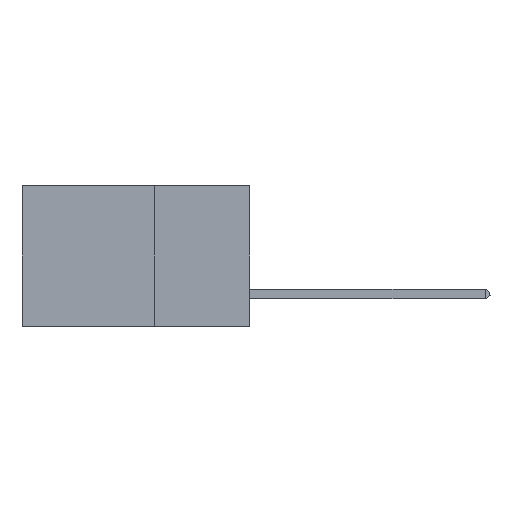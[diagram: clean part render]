
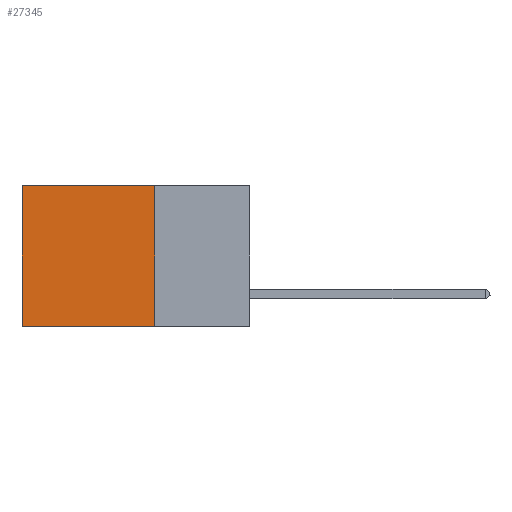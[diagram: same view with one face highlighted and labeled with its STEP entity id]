
A CAD part, left-side view. The second image highlights one B-rep face of the part: STEP entity #27345.
In plain terms, the highlighted planar face has unit normal (-1, 0, 0).
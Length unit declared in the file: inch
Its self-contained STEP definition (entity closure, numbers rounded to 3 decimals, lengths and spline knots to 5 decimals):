
#3004 = EDGE_CURVE ( 'NONE', #25553, #34495, #31278, .T. ) ;
#9082 = ORIENTED_EDGE ( 'NONE', *, *, #22281, .T. ) ;
#9734 = CARTESIAN_POINT ( 'NONE',  ( 0.2875, 0.25, 0. ) ) ;
#10029 = ORIENTED_EDGE ( 'NONE', *, *, #27524, .T. ) ;
#12877 = FACE_OUTER_BOUND ( 'NONE', #13228, .T. ) ;
#13228 = EDGE_LOOP ( 'NONE', ( #10029, #34841, #28919, #9082 ) ) ;
#13406 = VECTOR ( 'NONE', #40061, 39.37008 ) ;
#14698 = CARTESIAN_POINT ( 'NONE',  ( 0.2875, 0.25, -0.37 ) ) ;
#17171 = CARTESIAN_POINT ( 'NONE',  ( 0.2875, 0.6, -0.37 ) ) ;
#20604 = DIRECTION ( 'NONE',  ( 0., 1., 0. ) ) ;
#22114 = VECTOR ( 'NONE', #20604, 39.37008 ) ;
#22281 = EDGE_CURVE ( 'NONE', #36832, #34794, #28862, .T. ) ;
#22509 = LINE ( 'NONE', #36580, #13406 ) ;
#23322 = CARTESIAN_POINT ( 'NONE',  ( 0.2875, 0.25, -0.37 ) ) ;
#23557 = DIRECTION ( 'NONE',  ( 0., 1., 0. ) ) ;
#24412 = LINE ( 'NONE', #42494, #33559 ) ;
#25553 = VERTEX_POINT ( 'NONE', #14698 ) ;
#26775 = VECTOR ( 'NONE', #23557, 39.37008 ) ;
#27345 = ADVANCED_FACE ( 'NONE', ( #12877 ), #30386, .F. ) ;
#27524 = EDGE_CURVE ( 'NONE', #34794, #34495, #22509, .T. ) ;
#28862 = LINE ( 'NONE', #30308, #26775 ) ;
#28919 = ORIENTED_EDGE ( 'NONE', *, *, #34675, .F. ) ;
#29230 = AXIS2_PLACEMENT_3D ( 'NONE', #40011, #43619, #37605 ) ;
#29430 = CARTESIAN_POINT ( 'NONE',  ( 0.2875, 0.6, 0. ) ) ;
#30308 = CARTESIAN_POINT ( 'NONE',  ( 0.2875, 0.25, 0. ) ) ;
#30386 = PLANE ( 'NONE',  #29230 ) ;
#31278 = LINE ( 'NONE', #23322, #22114 ) ;
#32252 = DIRECTION ( 'NONE',  ( 0., 0., -1. ) ) ;
#33559 = VECTOR ( 'NONE', #32252, 39.37008 ) ;
#34495 = VERTEX_POINT ( 'NONE', #17171 ) ;
#34675 = EDGE_CURVE ( 'NONE', #36832, #25553, #24412, .T. ) ;
#34794 = VERTEX_POINT ( 'NONE', #29430 ) ;
#34841 = ORIENTED_EDGE ( 'NONE', *, *, #3004, .F. ) ;
#36580 = CARTESIAN_POINT ( 'NONE',  ( 0.2875, 0.6, 0. ) ) ;
#36832 = VERTEX_POINT ( 'NONE', #9734 ) ;
#37605 = DIRECTION ( 'NONE',  ( 0., 0., -1. ) ) ;
#40011 = CARTESIAN_POINT ( 'NONE',  ( 0.2875, 0.25, 0. ) ) ;
#40061 = DIRECTION ( 'NONE',  ( 0., 0., -1. ) ) ;
#42494 = CARTESIAN_POINT ( 'NONE',  ( 0.2875, 0.25, 0. ) ) ;
#43619 = DIRECTION ( 'NONE',  ( 1., 0., 0. ) ) ;
